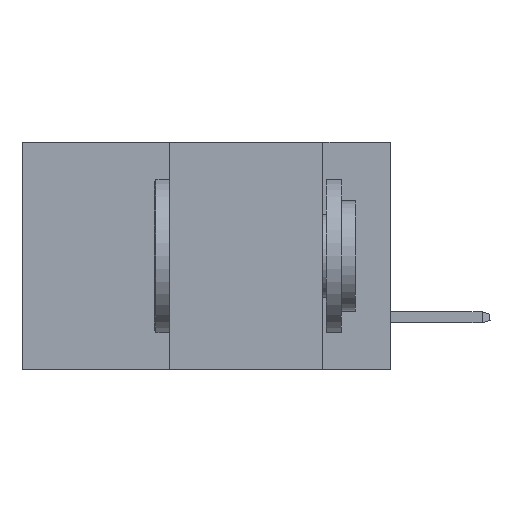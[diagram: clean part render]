
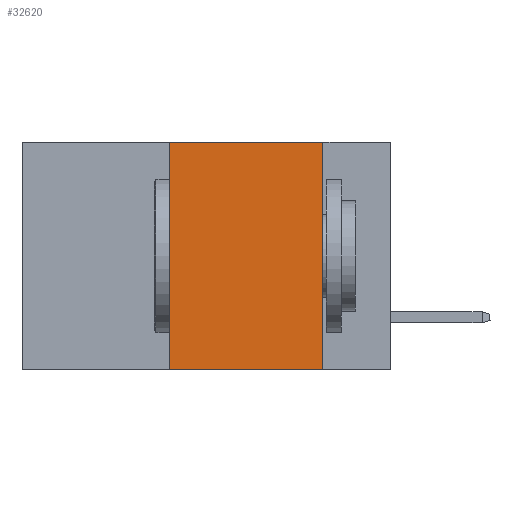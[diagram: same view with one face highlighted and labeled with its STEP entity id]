
A CAD part, left-side view. The second image highlights one B-rep face of the part: STEP entity #32620.
In plain terms, the highlighted planar face has unit normal (-1, 0, 0).
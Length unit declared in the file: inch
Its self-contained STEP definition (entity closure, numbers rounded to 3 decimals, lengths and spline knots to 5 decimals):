
#168 = VECTOR ( 'NONE', #22508, 39.37008 ) ;
#742 = DIRECTION ( 'NONE',  ( 0., -1., 0. ) ) ;
#1726 = CARTESIAN_POINT ( 'NONE',  ( 0., 0.6, 0. ) ) ;
#3760 = CARTESIAN_POINT ( 'NONE',  ( 0., 0.36, 0. ) ) ;
#3866 = CARTESIAN_POINT ( 'NONE',  ( 0., 0.6, -0.37 ) ) ;
#4018 = DIRECTION ( 'NONE',  ( 0., 0., 1. ) ) ;
#6881 = LINE ( 'NONE', #31908, #30838 ) ;
#9630 = VERTEX_POINT ( 'NONE', #15280 ) ;
#10207 = CARTESIAN_POINT ( 'NONE',  ( 0., 0.11, 0. ) ) ;
#12831 = EDGE_CURVE ( 'NONE', #34610, #30064, #23117, .T. ) ;
#15280 = CARTESIAN_POINT ( 'NONE',  ( 0., 0.36, -0.37 ) ) ;
#17512 = EDGE_CURVE ( 'NONE', #9630, #30064, #32418, .T. ) ;
#18383 = EDGE_LOOP ( 'NONE', ( #30005, #25251, #26815, #29609 ) ) ;
#20265 = DIRECTION ( 'NONE',  ( 1., 0., 0. ) ) ;
#21783 = VERTEX_POINT ( 'NONE', #3760 ) ;
#22508 = DIRECTION ( 'NONE',  ( 0., 0., -1. ) ) ;
#22713 = LINE ( 'NONE', #1726, #36924 ) ;
#23117 = LINE ( 'NONE', #10207, #168 ) ;
#24646 = FACE_OUTER_BOUND ( 'NONE', #18383, .T. ) ;
#24902 = EDGE_CURVE ( 'NONE', #9630, #21783, #6881, .T. ) ;
#25251 = ORIENTED_EDGE ( 'NONE', *, *, #26782, .F. ) ;
#26307 = AXIS2_PLACEMENT_3D ( 'NONE', #39289, #20265, #39571 ) ;
#26782 = EDGE_CURVE ( 'NONE', #21783, #34610, #22713, .T. ) ;
#26815 = ORIENTED_EDGE ( 'NONE', *, *, #24902, .F. ) ;
#27198 = DIRECTION ( 'NONE',  ( 0., -1., 0. ) ) ;
#29609 = ORIENTED_EDGE ( 'NONE', *, *, #17512, .T. ) ;
#30005 = ORIENTED_EDGE ( 'NONE', *, *, #12831, .F. ) ;
#30064 = VERTEX_POINT ( 'NONE', #35266 ) ;
#30118 = PLANE ( 'NONE',  #26307 ) ;
#30519 = CARTESIAN_POINT ( 'NONE',  ( 0., 0.11, 0. ) ) ;
#30838 = VECTOR ( 'NONE', #4018, 39.37008 ) ;
#31908 = CARTESIAN_POINT ( 'NONE',  ( 0., 0.36, 0. ) ) ;
#32418 = LINE ( 'NONE', #3866, #38792 ) ;
#32620 = ADVANCED_FACE ( 'NONE', ( #24646 ), #30118, .F. ) ;
#34610 = VERTEX_POINT ( 'NONE', #30519 ) ;
#35266 = CARTESIAN_POINT ( 'NONE',  ( 0., 0.11, -0.37 ) ) ;
#36924 = VECTOR ( 'NONE', #27198, 39.37008 ) ;
#38792 = VECTOR ( 'NONE', #742, 39.37008 ) ;
#39289 = CARTESIAN_POINT ( 'NONE',  ( 0., 0.6, 0. ) ) ;
#39571 = DIRECTION ( 'NONE',  ( 0., 0., -1. ) ) ;
